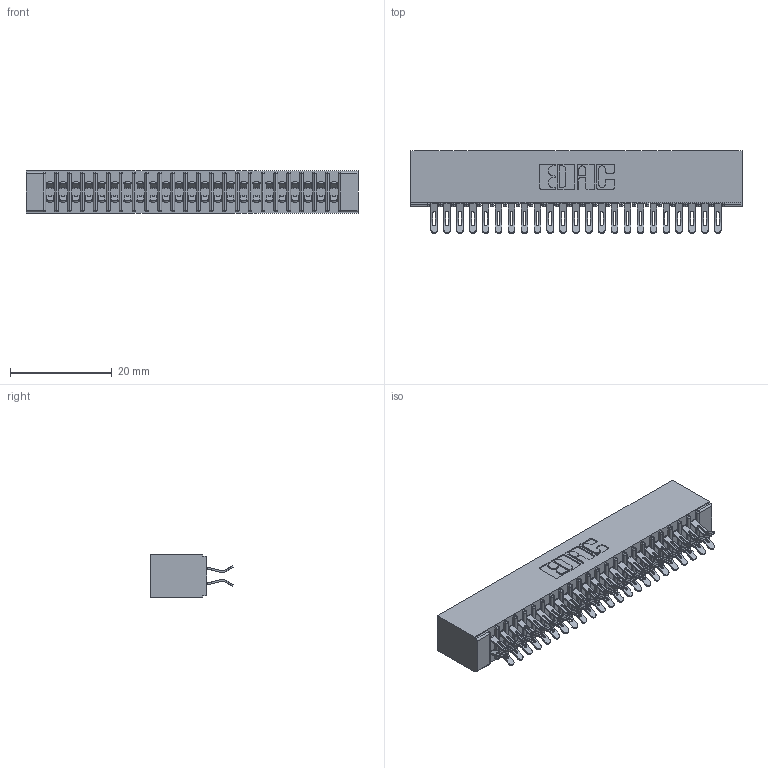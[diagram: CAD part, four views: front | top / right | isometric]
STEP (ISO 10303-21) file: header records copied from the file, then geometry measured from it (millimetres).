
FILE_DESCRIPTION (( 'STEP AP203' ), '1' );
FILE_NAME ('341-046-555-201.STEP', '2018-08-07T11:09:26', ( '' ), ( '' ), 'SwSTEP 2.0', 'SolidWorks 2016', '' );
FILE_SCHEMA (( 'CONFIG_CONTROL_DESIGN' ));
Length unit declared in the file: inch
Products named in the file (3): 341-292-001_341-292-155; 341-046-555-201; 341 Part_No Mounting Lugs
Assembly tree (47 placements, depth 2):
  341-046-555-201
    341 Part_No Mounting Lugs
    341-292-001_341-292-155  x46
Bounding box: 65.41 x 16.31 x 8.38 mm (x, y, z)
Volume: 3908.1 mm3; surface area: 9234.8 mm2
Topology: 47 solids, 47 shells, 3696 faces, 11033 edges, 7182 vertices
Faces by surface type: plane 1996, cylinder 1608, sphere 48, torus 44
Entity records: 30558 total; most frequent: CARTESIAN_POINT 5095, ORIENTED_EDGE 5050, DIRECTION 4947, EDGE_CURVE 2525, VECTOR 2007, LINE 2007, VERTEX_POINT 1602, AXIS2_PLACEMENT_3D 1470
